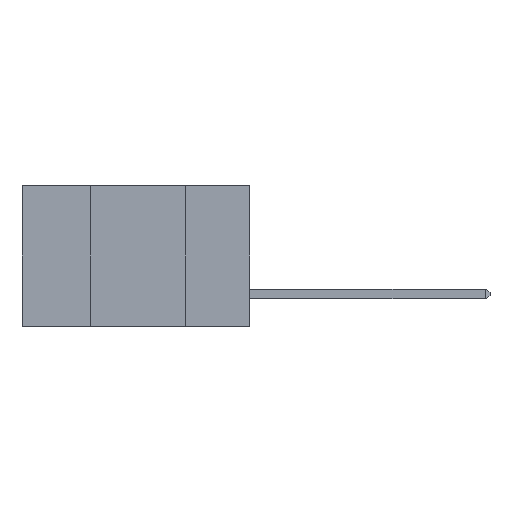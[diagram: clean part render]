
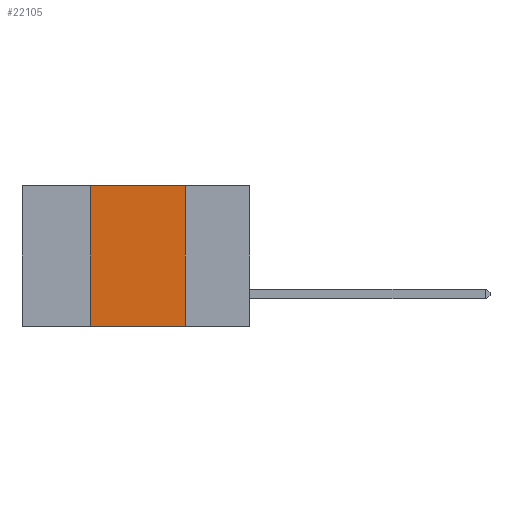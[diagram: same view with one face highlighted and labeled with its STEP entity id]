
A CAD part, left-side view. The second image highlights one B-rep face of the part: STEP entity #22105.
In plain terms, the highlighted planar face has unit normal (-1, 0, 0).
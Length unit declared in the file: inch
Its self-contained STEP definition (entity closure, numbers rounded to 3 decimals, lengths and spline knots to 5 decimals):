
#140 = CARTESIAN_POINT ( 'NONE',  ( 0., 0.17, 0. ) ) ;
#167 = ORIENTED_EDGE ( 'NONE', *, *, #23868, .T. ) ;
#347 = LINE ( 'NONE', #11160, #8111 ) ;
#1308 = ORIENTED_EDGE ( 'NONE', *, *, #1499, .F. ) ;
#1499 = EDGE_CURVE ( 'NONE', #14163, #35694, #9329, .T. ) ;
#1718 = CARTESIAN_POINT ( 'NONE',  ( 0., 0.6, 0. ) ) ;
#2877 = CARTESIAN_POINT ( 'NONE',  ( 0., 0.6, 0. ) ) ;
#5058 = DIRECTION ( 'NONE',  ( 0., 0., -1. ) ) ;
#5929 = VECTOR ( 'NONE', #6191, 39.37008 ) ;
#6191 = DIRECTION ( 'NONE',  ( 0., -1., 0. ) ) ;
#8111 = VECTOR ( 'NONE', #36206, 39.37008 ) ;
#8266 = LINE ( 'NONE', #18632, #40608 ) ;
#9329 = LINE ( 'NONE', #40649, #16764 ) ;
#11160 = CARTESIAN_POINT ( 'NONE',  ( 0., 0.42, 0. ) ) ;
#14163 = VERTEX_POINT ( 'NONE', #140 ) ;
#15132 = ORIENTED_EDGE ( 'NONE', *, *, #22582, .F. ) ;
#15380 = DIRECTION ( 'NONE',  ( 0., -1., 0. ) ) ;
#15389 = FACE_OUTER_BOUND ( 'NONE', #40854, .T. ) ;
#16764 = VECTOR ( 'NONE', #25294, 39.37008 ) ;
#18632 = CARTESIAN_POINT ( 'NONE',  ( 0., 0.6, -0.37 ) ) ;
#21111 = CARTESIAN_POINT ( 'NONE',  ( 0., 0.42, 0. ) ) ;
#22105 = ADVANCED_FACE ( 'NONE', ( #15389 ), #36526, .F. ) ;
#22582 = EDGE_CURVE ( 'NONE', #39694, #14163, #22904, .T. ) ;
#22739 = VERTEX_POINT ( 'NONE', #28930 ) ;
#22904 = LINE ( 'NONE', #2877, #5929 ) ;
#23868 = EDGE_CURVE ( 'NONE', #22739, #35694, #8266, .T. ) ;
#24201 = DIRECTION ( 'NONE',  ( 1., 0., 0. ) ) ;
#25294 = DIRECTION ( 'NONE',  ( 0., 0., -1. ) ) ;
#25987 = EDGE_CURVE ( 'NONE', #22739, #39694, #347, .T. ) ;
#28930 = CARTESIAN_POINT ( 'NONE',  ( 0., 0.42, -0.37 ) ) ;
#32958 = ORIENTED_EDGE ( 'NONE', *, *, #25987, .F. ) ;
#33721 = AXIS2_PLACEMENT_3D ( 'NONE', #1718, #24201, #5058 ) ;
#35694 = VERTEX_POINT ( 'NONE', #39981 ) ;
#36206 = DIRECTION ( 'NONE',  ( 0., 0., 1. ) ) ;
#36526 = PLANE ( 'NONE',  #33721 ) ;
#39694 = VERTEX_POINT ( 'NONE', #21111 ) ;
#39981 = CARTESIAN_POINT ( 'NONE',  ( 0., 0.17, -0.37 ) ) ;
#40608 = VECTOR ( 'NONE', #15380, 39.37008 ) ;
#40649 = CARTESIAN_POINT ( 'NONE',  ( 0., 0.17, 0. ) ) ;
#40854 = EDGE_LOOP ( 'NONE', ( #1308, #15132, #32958, #167 ) ) ;
